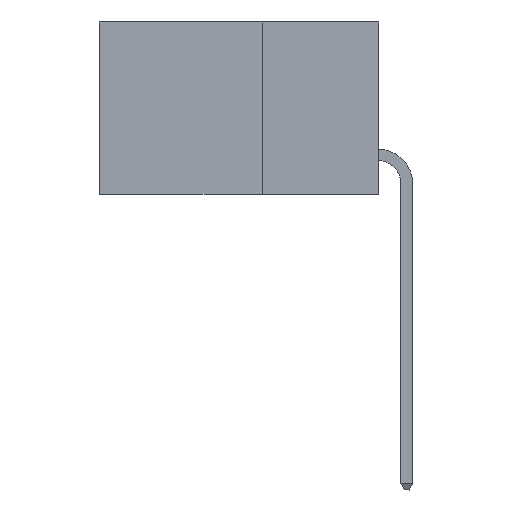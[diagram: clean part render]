
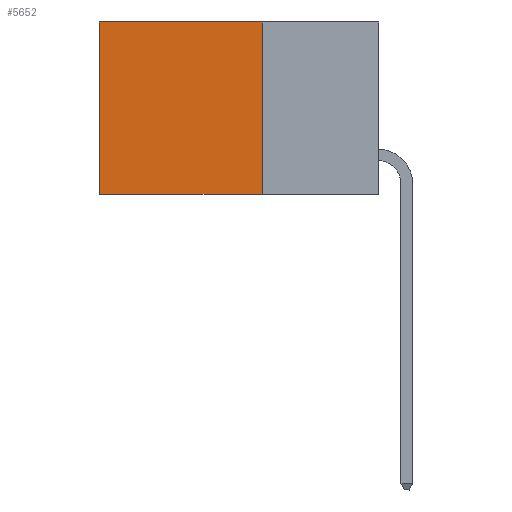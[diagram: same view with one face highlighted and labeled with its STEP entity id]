
A CAD part, left-side view. The second image highlights one B-rep face of the part: STEP entity #5652.
In plain terms, the highlighted planar face has unit normal (-1, 0, 0).
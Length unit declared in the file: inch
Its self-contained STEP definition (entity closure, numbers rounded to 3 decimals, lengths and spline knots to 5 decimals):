
#22 = VERTEX_POINT ( 'NONE', #1626 ) ;
#624 = DIRECTION ( 'NONE',  ( 0., 0., -1. ) ) ;
#697 = EDGE_CURVE ( 'NONE', #6858, #22, #6733, .T. ) ;
#1160 = CARTESIAN_POINT ( 'NONE',  ( 0.2615, 0.25, -0.37 ) ) ;
#1289 = DIRECTION ( 'NONE',  ( 0., 1., 0. ) ) ;
#1626 = CARTESIAN_POINT ( 'NONE',  ( 0.2615, 0.6, -0.37 ) ) ;
#1690 = VECTOR ( 'NONE', #624, 39.37008 ) ;
#2786 = CARTESIAN_POINT ( 'NONE',  ( 0.2615, 0.25, -0.37 ) ) ;
#2884 = ORIENTED_EDGE ( 'NONE', *, *, #9977, .F. ) ;
#3119 = DIRECTION ( 'NONE',  ( 1., 0., 0. ) ) ;
#3557 = VERTEX_POINT ( 'NONE', #11603 ) ;
#3638 = LINE ( 'NONE', #2786, #8753 ) ;
#3685 = CARTESIAN_POINT ( 'NONE',  ( 0.2615, 0.25, 0. ) ) ;
#3708 = EDGE_CURVE ( 'NONE', #8771, #3557, #6483, .T. ) ;
#3805 = CARTESIAN_POINT ( 'NONE',  ( 0.2615, 0.25, 0. ) ) ;
#4186 = PLANE ( 'NONE',  #10022 ) ;
#4309 = VECTOR ( 'NONE', #9055, 39.37008 ) ;
#4445 = ORIENTED_EDGE ( 'NONE', *, *, #8623, .T. ) ;
#5418 = DIRECTION ( 'NONE',  ( 0., 0., -1. ) ) ;
#5652 = ADVANCED_FACE ( 'NONE', ( #6802 ), #4186, .F. ) ;
#6483 = LINE ( 'NONE', #3805, #4309 ) ;
#6733 = LINE ( 'NONE', #1160, #7334 ) ;
#6739 = DIRECTION ( 'NONE',  ( 0., 0., -1. ) ) ;
#6802 = FACE_OUTER_BOUND ( 'NONE', #10298, .T. ) ;
#6858 = VERTEX_POINT ( 'NONE', #9669 ) ;
#7334 = VECTOR ( 'NONE', #1289, 39.37008 ) ;
#7627 = CARTESIAN_POINT ( 'NONE',  ( 0.2615, 0.25, -0.37 ) ) ;
#7684 = ORIENTED_EDGE ( 'NONE', *, *, #697, .F. ) ;
#7803 = LINE ( 'NONE', #8812, #1690 ) ;
#8623 = EDGE_CURVE ( 'NONE', #3557, #22, #7803, .T. ) ;
#8753 = VECTOR ( 'NONE', #5418, 39.37008 ) ;
#8771 = VERTEX_POINT ( 'NONE', #3685 ) ;
#8812 = CARTESIAN_POINT ( 'NONE',  ( 0.2615, 0.6, -0.37 ) ) ;
#9055 = DIRECTION ( 'NONE',  ( 0., 1., 0. ) ) ;
#9669 = CARTESIAN_POINT ( 'NONE',  ( 0.2615, 0.25, -0.37 ) ) ;
#9977 = EDGE_CURVE ( 'NONE', #8771, #6858, #3638, .T. ) ;
#10022 = AXIS2_PLACEMENT_3D ( 'NONE', #7627, #3119, #6739 ) ;
#10298 = EDGE_LOOP ( 'NONE', ( #4445, #7684, #2884, #11266 ) ) ;
#11266 = ORIENTED_EDGE ( 'NONE', *, *, #3708, .T. ) ;
#11603 = CARTESIAN_POINT ( 'NONE',  ( 0.2615, 0.6, 0. ) ) ;
